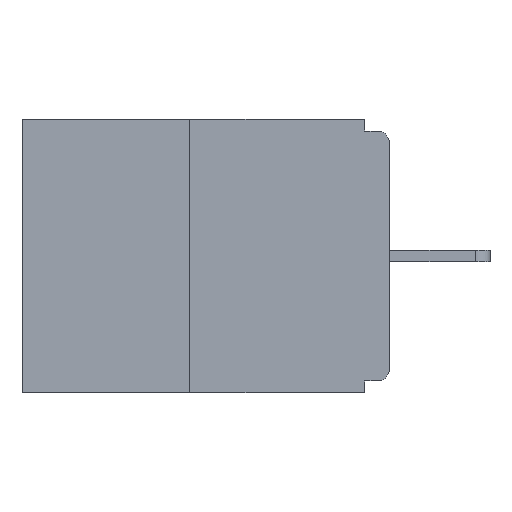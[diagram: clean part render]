
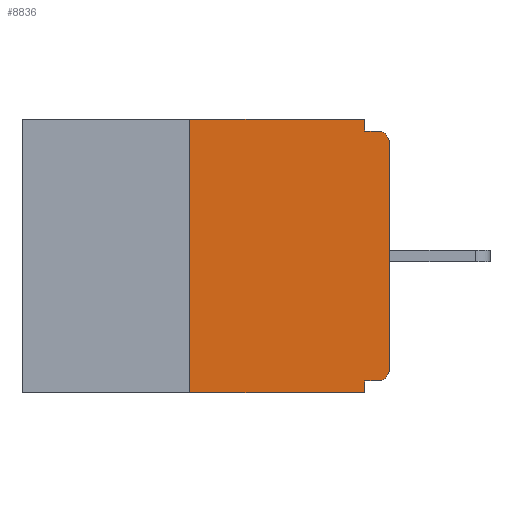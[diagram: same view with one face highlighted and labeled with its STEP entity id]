
A CAD part, left-side view. The second image highlights one B-rep face of the part: STEP entity #8836.
In plain terms, the highlighted planar face has unit normal (-1, 0, 0).
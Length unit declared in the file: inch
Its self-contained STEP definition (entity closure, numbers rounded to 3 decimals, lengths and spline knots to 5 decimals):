
#374 = DIRECTION ( 'NONE',  ( 0., 0., -1. ) ) ;
#429 = VERTEX_POINT ( 'NONE', #5686 ) ;
#441 = DIRECTION ( 'NONE',  ( 0., 0., 1. ) ) ;
#454 = ORIENTED_EDGE ( 'NONE', *, *, #6763, .F. ) ;
#688 = EDGE_CURVE ( 'NONE', #429, #4788, #13708, .T. ) ;
#810 = VECTOR ( 'NONE', #3961, 39.37008 ) ;
#1377 = VERTEX_POINT ( 'NONE', #2871 ) ;
#2562 = CARTESIAN_POINT ( 'NONE',  ( 0., 0.031, 0. ) ) ;
#2625 = DIRECTION ( 'NONE',  ( 0., 1., 0. ) ) ;
#2752 = DIRECTION ( 'NONE',  ( -1., 0., 0. ) ) ;
#2871 = CARTESIAN_POINT ( 'NONE',  ( 0., 0.25, 0. ) ) ;
#3709 = VERTEX_POINT ( 'NONE', #4075 ) ;
#3812 = LINE ( 'NONE', #12232, #810 ) ;
#3894 = VECTOR ( 'NONE', #8792, 39.37008 ) ;
#3961 = DIRECTION ( 'NONE',  ( 0., -1., 0. ) ) ;
#3984 = CARTESIAN_POINT ( 'NONE',  ( 0., 0.015, -0.313 ) ) ;
#4075 = CARTESIAN_POINT ( 'NONE',  ( 0., 0.031, -0.015 ) ) ;
#4163 = PLANE ( 'NONE',  #14808 ) ;
#4178 = LINE ( 'NONE', #10622, #13884 ) ;
#4292 = LINE ( 'NONE', #2562, #3894 ) ;
#4357 = VECTOR ( 'NONE', #2625, 39.37008 ) ;
#4614 = CARTESIAN_POINT ( 'NONE',  ( 0., 0., -0.328 ) ) ;
#4788 = VERTEX_POINT ( 'NONE', #8674 ) ;
#4963 = EDGE_CURVE ( 'NONE', #8855, #6726, #15252, .T. ) ;
#5233 = DIRECTION ( 'NONE',  ( 0., 0., -1. ) ) ;
#5539 = VERTEX_POINT ( 'NONE', #8731 ) ;
#5686 = CARTESIAN_POINT ( 'NONE',  ( 0., 0.015, -0.328 ) ) ;
#5922 = DIRECTION ( 'NONE',  ( 0., -1., 0. ) ) ;
#5976 = VERTEX_POINT ( 'NONE', #6216 ) ;
#5996 = VERTEX_POINT ( 'NONE', #6266 ) ;
#6096 = ORIENTED_EDGE ( 'NONE', *, *, #9893, .F. ) ;
#6135 = EDGE_CURVE ( 'NONE', #6726, #5976, #12433, .T. ) ;
#6216 = CARTESIAN_POINT ( 'NONE',  ( 0., 0.015, -0.015 ) ) ;
#6266 = CARTESIAN_POINT ( 'NONE',  ( 0., 0.031, -0.343 ) ) ;
#6396 = ORIENTED_EDGE ( 'NONE', *, *, #8387, .T. ) ;
#6400 = ORIENTED_EDGE ( 'NONE', *, *, #7567, .F. ) ;
#6511 = ORIENTED_EDGE ( 'NONE', *, *, #688, .F. ) ;
#6578 = ORIENTED_EDGE ( 'NONE', *, *, #9348, .T. ) ;
#6726 = VERTEX_POINT ( 'NONE', #14311 ) ;
#6727 = DIRECTION ( 'NONE',  ( 0., 0., -1. ) ) ;
#6763 = EDGE_CURVE ( 'NONE', #11774, #3709, #4292, .T. ) ;
#6809 = ORIENTED_EDGE ( 'NONE', *, *, #9978, .F. ) ;
#6842 = ORIENTED_EDGE ( 'NONE', *, *, #10837, .F. ) ;
#7169 = ORIENTED_EDGE ( 'NONE', *, *, #6135, .T. ) ;
#7212 = VECTOR ( 'NONE', #10760, 39.37008 ) ;
#7567 = EDGE_CURVE ( 'NONE', #4788, #5996, #8923, .T. ) ;
#7946 = DIRECTION ( 'NONE',  ( 1., 0., 0. ) ) ;
#8111 = EDGE_LOOP ( 'NONE', ( #6809, #6096, #6396, #6400, #6511, #6578, #10440, #7169, #6842, #454 ) ) ;
#8387 = EDGE_CURVE ( 'NONE', #5539, #5996, #13257, .T. ) ;
#8674 = CARTESIAN_POINT ( 'NONE',  ( 0., 0.031, -0.328 ) ) ;
#8731 = CARTESIAN_POINT ( 'NONE',  ( 0., 0.25, -0.343 ) ) ;
#8792 = DIRECTION ( 'NONE',  ( 0., 0., -1. ) ) ;
#8836 = ADVANCED_FACE ( 'NONE', ( #10287 ), #4163, .F. ) ;
#8855 = VERTEX_POINT ( 'NONE', #9104 ) ;
#8923 = LINE ( 'NONE', #13572, #14868 ) ;
#9071 = AXIS2_PLACEMENT_3D ( 'NONE', #10033, #2752, #11156 ) ;
#9104 = CARTESIAN_POINT ( 'NONE',  ( 0., 0., -0.313 ) ) ;
#9348 = EDGE_CURVE ( 'NONE', #429, #8855, #9576, .T. ) ;
#9576 = CIRCLE ( 'NONE', #13494, 0.015 ) ;
#9658 = CARTESIAN_POINT ( 'NONE',  ( 0., 0.031, 0. ) ) ;
#9893 = EDGE_CURVE ( 'NONE', #5539, #1377, #14091, .T. ) ;
#9978 = EDGE_CURVE ( 'NONE', #1377, #11774, #3812, .T. ) ;
#10033 = CARTESIAN_POINT ( 'NONE',  ( 0., 0.015, -0.03 ) ) ;
#10184 = CARTESIAN_POINT ( 'NONE',  ( 0., 0.46, 0. ) ) ;
#10287 = FACE_OUTER_BOUND ( 'NONE', #8111, .T. ) ;
#10440 = ORIENTED_EDGE ( 'NONE', *, *, #4963, .T. ) ;
#10622 = CARTESIAN_POINT ( 'NONE',  ( 0., 0., -0.015 ) ) ;
#10760 = DIRECTION ( 'NONE',  ( 0., -1., 0. ) ) ;
#10837 = EDGE_CURVE ( 'NONE', #3709, #5976, #4178, .T. ) ;
#11128 = VECTOR ( 'NONE', #13216, 39.37008 ) ;
#11156 = DIRECTION ( 'NONE',  ( 0., 0., -1. ) ) ;
#11774 = VERTEX_POINT ( 'NONE', #9658 ) ;
#12084 = CARTESIAN_POINT ( 'NONE',  ( 0., 0.25, 0. ) ) ;
#12232 = CARTESIAN_POINT ( 'NONE',  ( 0., 0.46, 0. ) ) ;
#12248 = DIRECTION ( 'NONE',  ( -1., 0., 0. ) ) ;
#12433 = CIRCLE ( 'NONE', #9071, 0.015 ) ;
#13216 = DIRECTION ( 'NONE',  ( 0., 0., 1. ) ) ;
#13257 = LINE ( 'NONE', #14080, #7212 ) ;
#13494 = AXIS2_PLACEMENT_3D ( 'NONE', #3984, #12248, #5233 ) ;
#13572 = CARTESIAN_POINT ( 'NONE',  ( 0., 0.031, -0.343 ) ) ;
#13708 = LINE ( 'NONE', #4614, #4357 ) ;
#13884 = VECTOR ( 'NONE', #5922, 39.37008 ) ;
#14080 = CARTESIAN_POINT ( 'NONE',  ( 0., 0.46, -0.343 ) ) ;
#14091 = LINE ( 'NONE', #12084, #11128 ) ;
#14255 = CARTESIAN_POINT ( 'NONE',  ( 0., 0., 0. ) ) ;
#14311 = CARTESIAN_POINT ( 'NONE',  ( 0., 0., -0.03 ) ) ;
#14808 = AXIS2_PLACEMENT_3D ( 'NONE', #10184, #7946, #374 ) ;
#14868 = VECTOR ( 'NONE', #6727, 39.37008 ) ;
#14918 = VECTOR ( 'NONE', #441, 39.37008 ) ;
#15252 = LINE ( 'NONE', #14255, #14918 ) ;
